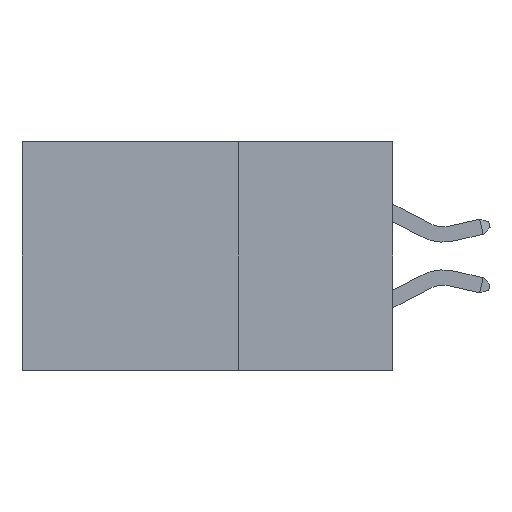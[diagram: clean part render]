
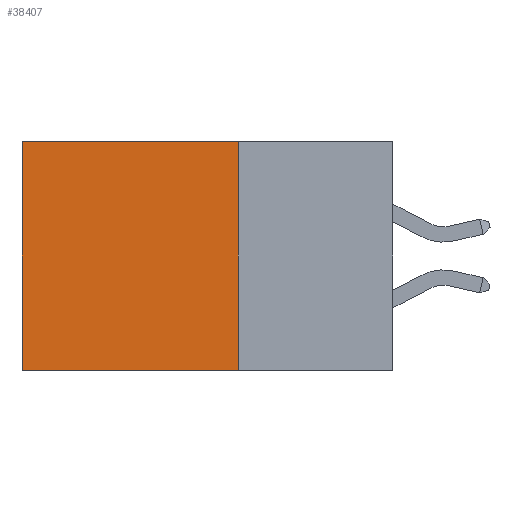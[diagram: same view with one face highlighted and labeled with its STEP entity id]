
A CAD part, left-side view. The second image highlights one B-rep face of the part: STEP entity #38407.
In plain terms, the highlighted planar face has unit normal (-1, 0, 0).
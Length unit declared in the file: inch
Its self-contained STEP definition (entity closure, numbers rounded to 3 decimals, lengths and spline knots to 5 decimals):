
#824 = EDGE_CURVE ( 'NONE', #42489, #901, #32502, .T. ) ;
#901 = VERTEX_POINT ( 'NONE', #16229 ) ;
#1993 = CARTESIAN_POINT ( 'NONE',  ( 0.2875, 0.6, -0.37 ) ) ;
#6895 = ORIENTED_EDGE ( 'NONE', *, *, #30527, .F. ) ;
#7169 = DIRECTION ( 'NONE',  ( 0., 1., 0. ) ) ;
#10367 = VECTOR ( 'NONE', #15670, 39.37008 ) ;
#10677 = LINE ( 'NONE', #34616, #19019 ) ;
#12178 = FACE_OUTER_BOUND ( 'NONE', #33506, .T. ) ;
#15209 = CARTESIAN_POINT ( 'NONE',  ( 0.2875, 0.25, 0. ) ) ;
#15670 = DIRECTION ( 'NONE',  ( 0., 0., -1. ) ) ;
#16229 = CARTESIAN_POINT ( 'NONE',  ( 0.2875, 0.6, 0. ) ) ;
#16646 = CARTESIAN_POINT ( 'NONE',  ( 0.2875, 0.25, 0. ) ) ;
#16730 = VECTOR ( 'NONE', #43249, 39.37008 ) ;
#17505 = EDGE_CURVE ( 'NONE', #901, #43184, #29193, .T. ) ;
#18039 = ORIENTED_EDGE ( 'NONE', *, *, #17505, .T. ) ;
#18522 = LINE ( 'NONE', #15209, #10367 ) ;
#19019 = VECTOR ( 'NONE', #7169, 39.37008 ) ;
#20720 = ORIENTED_EDGE ( 'NONE', *, *, #24257, .F. ) ;
#22506 = PLANE ( 'NONE',  #25475 ) ;
#24257 = EDGE_CURVE ( 'NONE', #24357, #43184, #10677, .T. ) ;
#24357 = VERTEX_POINT ( 'NONE', #30872 ) ;
#25475 = AXIS2_PLACEMENT_3D ( 'NONE', #36336, #25789, #32817 ) ;
#25789 = DIRECTION ( 'NONE',  ( 1., 0., 0. ) ) ;
#26334 = CARTESIAN_POINT ( 'NONE',  ( 0.2875, 0.6, 0. ) ) ;
#29193 = LINE ( 'NONE', #26334, #35243 ) ;
#29840 = ORIENTED_EDGE ( 'NONE', *, *, #824, .T. ) ;
#30527 = EDGE_CURVE ( 'NONE', #42489, #24357, #18522, .T. ) ;
#30872 = CARTESIAN_POINT ( 'NONE',  ( 0.2875, 0.25, -0.37 ) ) ;
#32502 = LINE ( 'NONE', #35796, #16730 ) ;
#32817 = DIRECTION ( 'NONE',  ( 0., 0., -1. ) ) ;
#33506 = EDGE_LOOP ( 'NONE', ( #18039, #20720, #6895, #29840 ) ) ;
#34616 = CARTESIAN_POINT ( 'NONE',  ( 0.2875, 0.25, -0.37 ) ) ;
#35243 = VECTOR ( 'NONE', #39753, 39.37008 ) ;
#35796 = CARTESIAN_POINT ( 'NONE',  ( 0.2875, 0.25, 0. ) ) ;
#36336 = CARTESIAN_POINT ( 'NONE',  ( 0.2875, 0.25, 0. ) ) ;
#38407 = ADVANCED_FACE ( 'NONE', ( #12178 ), #22506, .F. ) ;
#39753 = DIRECTION ( 'NONE',  ( 0., 0., -1. ) ) ;
#42489 = VERTEX_POINT ( 'NONE', #16646 ) ;
#43184 = VERTEX_POINT ( 'NONE', #1993 ) ;
#43249 = DIRECTION ( 'NONE',  ( 0., 1., 0. ) ) ;
